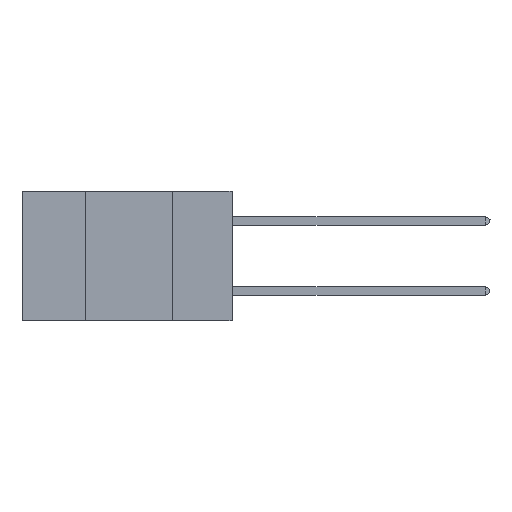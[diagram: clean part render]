
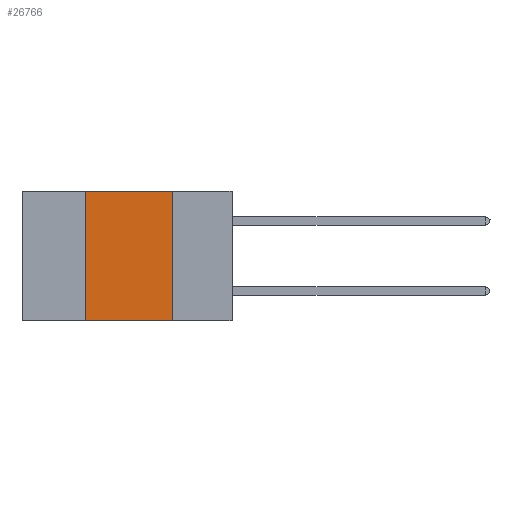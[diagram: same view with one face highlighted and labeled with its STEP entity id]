
A CAD part, left-side view. The second image highlights one B-rep face of the part: STEP entity #26766.
In plain terms, the highlighted planar face has unit normal (-1, 0, 0).
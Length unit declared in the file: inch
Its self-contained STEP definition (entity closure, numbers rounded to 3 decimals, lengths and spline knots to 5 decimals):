
#301 = CARTESIAN_POINT ( 'NONE',  ( 0., 0.6, 0. ) ) ;
#1414 = LINE ( 'NONE', #22219, #2091 ) ;
#1714 = ORIENTED_EDGE ( 'NONE', *, *, #6255, .F. ) ;
#2091 = VECTOR ( 'NONE', #11799, 39.37008 ) ;
#2132 = CARTESIAN_POINT ( 'NONE',  ( 0., 0.42, 0. ) ) ;
#3357 = EDGE_CURVE ( 'NONE', #24765, #20388, #1414, .T. ) ;
#4304 = ORIENTED_EDGE ( 'NONE', *, *, #16523, .F. ) ;
#4564 = DIRECTION ( 'NONE',  ( 0., -1., 0. ) ) ;
#6255 = EDGE_CURVE ( 'NONE', #26711, #24765, #16245, .T. ) ;
#7457 = EDGE_LOOP ( 'NONE', ( #25718, #1714, #4304, #23667 ) ) ;
#8363 = PLANE ( 'NONE',  #20090 ) ;
#9172 = LINE ( 'NONE', #2132, #23721 ) ;
#11012 = CARTESIAN_POINT ( 'NONE',  ( 0., 0.17, -0.37 ) ) ;
#11145 = VERTEX_POINT ( 'NONE', #24911 ) ;
#11184 = FACE_OUTER_BOUND ( 'NONE', #7457, .T. ) ;
#11799 = DIRECTION ( 'NONE',  ( 0., 0., -1. ) ) ;
#11910 = CARTESIAN_POINT ( 'NONE',  ( 0., 0.17, 0. ) ) ;
#12260 = DIRECTION ( 'NONE',  ( 0., 0., -1. ) ) ;
#14859 = VECTOR ( 'NONE', #15091, 39.37008 ) ;
#15091 = DIRECTION ( 'NONE',  ( 0., -1., 0. ) ) ;
#15245 = EDGE_CURVE ( 'NONE', #11145, #20388, #24785, .T. ) ;
#16245 = LINE ( 'NONE', #301, #26210 ) ;
#16523 = EDGE_CURVE ( 'NONE', #11145, #26711, #9172, .T. ) ;
#16649 = DIRECTION ( 'NONE',  ( 1., 0., 0. ) ) ;
#18598 = CARTESIAN_POINT ( 'NONE',  ( 0., 0.6, 0. ) ) ;
#20090 = AXIS2_PLACEMENT_3D ( 'NONE', #18598, #16649, #12260 ) ;
#20388 = VERTEX_POINT ( 'NONE', #11012 ) ;
#21365 = CARTESIAN_POINT ( 'NONE',  ( 0., 0.6, -0.37 ) ) ;
#22219 = CARTESIAN_POINT ( 'NONE',  ( 0., 0.17, 0. ) ) ;
#22864 = CARTESIAN_POINT ( 'NONE',  ( 0., 0.42, 0. ) ) ;
#23302 = DIRECTION ( 'NONE',  ( 0., 0., 1. ) ) ;
#23667 = ORIENTED_EDGE ( 'NONE', *, *, #15245, .T. ) ;
#23721 = VECTOR ( 'NONE', #23302, 39.37008 ) ;
#24765 = VERTEX_POINT ( 'NONE', #11910 ) ;
#24785 = LINE ( 'NONE', #21365, #14859 ) ;
#24911 = CARTESIAN_POINT ( 'NONE',  ( 0., 0.42, -0.37 ) ) ;
#25718 = ORIENTED_EDGE ( 'NONE', *, *, #3357, .F. ) ;
#26210 = VECTOR ( 'NONE', #4564, 39.37008 ) ;
#26711 = VERTEX_POINT ( 'NONE', #22864 ) ;
#26766 = ADVANCED_FACE ( 'NONE', ( #11184 ), #8363, .F. ) ;
